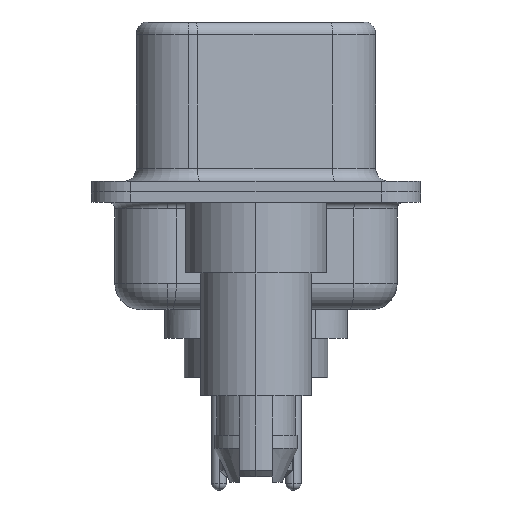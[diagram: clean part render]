
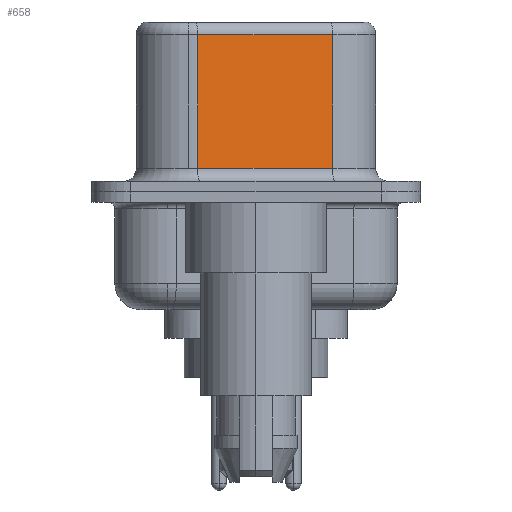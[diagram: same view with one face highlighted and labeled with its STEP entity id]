
A CAD part, left-side view. The second image highlights one B-rep face of the part: STEP entity #658.
In plain terms, the highlighted planar face has unit normal (-0.985, -0.174, 0).
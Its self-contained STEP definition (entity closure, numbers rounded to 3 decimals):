
#364 = CARTESIAN_POINT ( 'NONE',  ( 4.565, -2.927, 0.9 ) ) ;
#658 = ADVANCED_FACE ( 'NONE', ( #7848 ), #9267, .F. ) ;
#1038 = VECTOR ( 'NONE', #14738, 1000. ) ;
#1129 = EDGE_CURVE ( 'NONE', #14592, #19986, #11415, .T. ) ;
#1270 = EDGE_CURVE ( 'NONE', #12521, #6194, #1556, .T. ) ;
#1291 = EDGE_CURVE ( 'NONE', #12521, #19986, #13174, .T. ) ;
#1556 = LINE ( 'NONE', #12281, #1038 ) ;
#2426 = ORIENTED_EDGE ( 'NONE', *, *, #1291, .F. ) ;
#3417 = CARTESIAN_POINT ( 'NONE',  ( 3.655, 2.233, 6.02 ) ) ;
#4293 = ORIENTED_EDGE ( 'NONE', *, *, #1270, .T. ) ;
#5887 = CARTESIAN_POINT ( 'NONE',  ( 4.565, -2.927, 6.52 ) ) ;
#6194 = VERTEX_POINT ( 'NONE', #3417 ) ;
#7848 = FACE_OUTER_BOUND ( 'NONE', #16146, .T. ) ;
#8273 = LINE ( 'NONE', #18817, #10442 ) ;
#9022 = VECTOR ( 'NONE', #9356, 1000. ) ;
#9267 = PLANE ( 'NONE',  #16164 ) ;
#9356 = DIRECTION ( 'NONE',  ( 0., 0., -1. ) ) ;
#10442 = VECTOR ( 'NONE', #12261, 1000. ) ;
#11415 = LINE ( 'NONE', #15140, #19549 ) ;
#12066 = ORIENTED_EDGE ( 'NONE', *, *, #1129, .T. ) ;
#12261 = DIRECTION ( 'NONE',  ( 0., 0., -1. ) ) ;
#12281 = CARTESIAN_POINT ( 'NONE',  ( 4.565, -2.927, 6.02 ) ) ;
#12521 = VERTEX_POINT ( 'NONE', #19879 ) ;
#13174 = LINE ( 'NONE', #17710, #9022 ) ;
#14380 = CARTESIAN_POINT ( 'NONE',  ( 3.655, 2.233, 0.9 ) ) ;
#14592 = VERTEX_POINT ( 'NONE', #14380 ) ;
#14738 = DIRECTION ( 'NONE',  ( -0.174, 0.985, 0. ) ) ;
#15108 = ORIENTED_EDGE ( 'NONE', *, *, #16265, .T. ) ;
#15140 = CARTESIAN_POINT ( 'NONE',  ( 4.565, -2.927, 0.9 ) ) ;
#16146 = EDGE_LOOP ( 'NONE', ( #2426, #4293, #15108, #12066 ) ) ;
#16164 = AXIS2_PLACEMENT_3D ( 'NONE', #5887, #20512, #19516 ) ;
#16265 = EDGE_CURVE ( 'NONE', #6194, #14592, #8273, .T. ) ;
#17710 = CARTESIAN_POINT ( 'NONE',  ( 4.565, -2.927, 6.52 ) ) ;
#18590 = DIRECTION ( 'NONE',  ( 0.174, -0.985, 0. ) ) ;
#18817 = CARTESIAN_POINT ( 'NONE',  ( 3.655, 2.233, 6.52 ) ) ;
#19516 = DIRECTION ( 'NONE',  ( -0.174, 0.985, 0. ) ) ;
#19549 = VECTOR ( 'NONE', #18590, 1000. ) ;
#19879 = CARTESIAN_POINT ( 'NONE',  ( 4.565, -2.927, 6.02 ) ) ;
#19986 = VERTEX_POINT ( 'NONE', #364 ) ;
#20512 = DIRECTION ( 'NONE',  ( 0.985, 0.174, 0. ) ) ;
